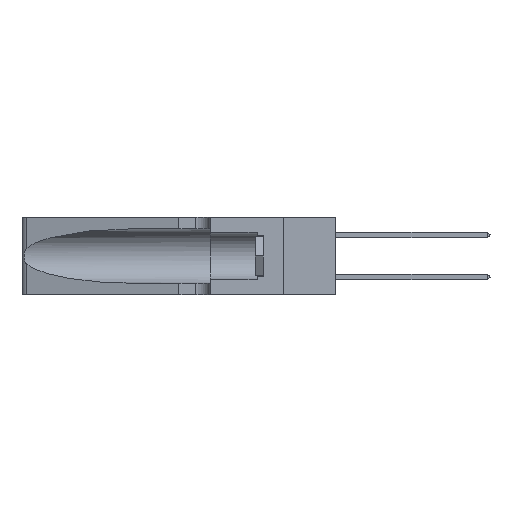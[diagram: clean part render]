
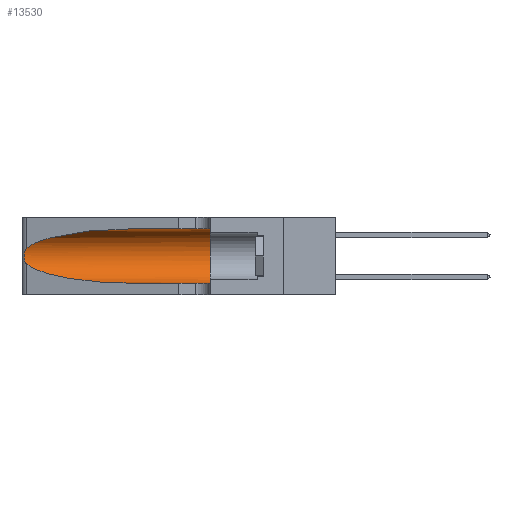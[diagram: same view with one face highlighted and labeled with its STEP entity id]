
A CAD part, left-side view. The second image highlights one B-rep face of the part: STEP entity #13530.
In plain terms, the highlighted cylindrical face has radius 3.308 mm (diameter 6.617 mm), a partial arc.
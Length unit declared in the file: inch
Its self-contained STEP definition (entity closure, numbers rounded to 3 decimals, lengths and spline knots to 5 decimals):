
#371 = CARTESIAN_POINT ( 'NONE',  ( 0.25487, 1.22718, 0.14631 ) ) ;
#1066 = CARTESIAN_POINT ( 'NONE',  ( 0.1305, 0.35, 0.185 ) ) ;
#2398 = CARTESIAN_POINT ( 'NONE',  ( 0.25487, 1.22718, 0.14631 ) ) ;
#3431 = ORIENTED_EDGE ( 'NONE', *, *, #36711, .T. ) ;
#3549 = VERTEX_POINT ( 'NONE', #10067 ) ;
#3583 = CARTESIAN_POINT ( 'NONE',  ( 0.18966, 0.96281, 0.05475 ) ) ;
#4281 = DIRECTION ( 'NONE',  ( 0., 0., 1. ) ) ;
#5246 = CARTESIAN_POINT ( 'NONE',  ( 0.25787, 1.23484, 0.2124 ) ) ;
#6549 = AXIS2_PLACEMENT_3D ( 'NONE', #31095, #12127, #34267 ) ;
#7136 =( BOUNDED_CURVE ( )  B_SPLINE_CURVE ( 3, ( #371, #22571, #3583, #25763 ),
 .UNSPECIFIED., .F., .F. ) 
 B_SPLINE_CURVE_WITH_KNOTS ( ( 4, 4 ),
 ( 3.44316, 4.71239 ),
 .UNSPECIFIED. ) 
 CURVE ( )  GEOMETRIC_REPRESENTATION_ITEM ( )  RATIONAL_B_SPLINE_CURVE ( ( 1., 0.87, 0.87, 1. ) ) 
 REPRESENTATION_ITEM ( '' )  );
#7374 = CARTESIAN_POINT ( 'NONE',  ( 0.18966, 0.96281, 0.31525 ) ) ;
#7692 = VERTEX_POINT ( 'NONE', #39892 ) ;
#8450 = CARTESIAN_POINT ( 'NONE',  ( 0.26018, 1.23835, 0.19895 ) ) ;
#10067 = CARTESIAN_POINT ( 'NONE',  ( 0.1305, 0.35, 0.31525 ) ) ;
#10235 = EDGE_CURVE ( 'NONE', #15838, #3549, #18555, .T. ) ;
#10703 = CARTESIAN_POINT ( 'NONE',  ( 0.25487, 1.22718, 0.22369 ) ) ;
#11637 = CARTESIAN_POINT ( 'NONE',  ( 0.26075, 1.23896, 0.178 ) ) ;
#12127 = DIRECTION ( 'NONE',  ( 0., -1., 0. ) ) ;
#12201 = ORIENTED_EDGE ( 'NONE', *, *, #10235, .F. ) ;
#12465 = EDGE_CURVE ( 'NONE', #3549, #7692, #32204, .T. ) ;
#12592 = CARTESIAN_POINT ( 'NONE',  ( 0.1305, 0.72297, 0.05475 ) ) ;
#13333 = EDGE_CURVE ( 'NONE', #40776, #7692, #33110, .T. ) ;
#13474 = CARTESIAN_POINT ( 'NONE',  ( 0.1305, 1.61858, 0.31525 ) ) ;
#13530 = ADVANCED_FACE ( 'NONE', ( #17751 ), #33596, .F. ) ;
#13596 = ORIENTED_EDGE ( 'NONE', *, *, #12465, .F. ) ;
#14539 =( BOUNDED_CURVE ( )  B_SPLINE_CURVE ( 3, ( #32715, #7374, #29679, #10703 ),
 .UNSPECIFIED., .F., .F. ) 
 B_SPLINE_CURVE_WITH_KNOTS ( ( 4, 4 ),
 ( 1.5708, 2.84003 ),
 .UNSPECIFIED. ) 
 CURVE ( )  GEOMETRIC_REPRESENTATION_ITEM ( )  RATIONAL_B_SPLINE_CURVE ( ( 1., 0.87, 0.87, 1. ) ) 
 REPRESENTATION_ITEM ( '' )  );
#14837 = CARTESIAN_POINT ( 'NONE',  ( 0.25856, 1.23593, 0.16098 ) ) ;
#15320 = AXIS2_PLACEMENT_3D ( 'NONE', #1066, #23251, #4281 ) ;
#15533 = CARTESIAN_POINT ( 'NONE',  ( 0.25487, 1.22718, 0.22369 ) ) ;
#15838 = VERTEX_POINT ( 'NONE', #24839 ) ;
#16656 = DIRECTION ( 'NONE',  ( 0., -1., 0. ) ) ;
#17751 = FACE_OUTER_BOUND ( 'NONE', #33322, .T. ) ;
#17870 = CARTESIAN_POINT ( 'NONE',  ( 0.25487, 1.22718, 0.22369 ) ) ;
#18007 = CARTESIAN_POINT ( 'NONE',  ( 0.25639, 1.23186, 0.15144 ) ) ;
#18555 = LINE ( 'NONE', #13474, #33391 ) ;
#20905 = ORIENTED_EDGE ( 'NONE', *, *, #35336, .T. ) ;
#21173 = CARTESIAN_POINT ( 'NONE',  ( 0.25487, 1.22718, 0.14631 ) ) ;
#22571 = CARTESIAN_POINT ( 'NONE',  ( 0.2373, 1.15595, 0.08982 ) ) ;
#23251 = DIRECTION ( 'NONE',  ( 0., 1., 0. ) ) ;
#23894 = DIRECTION ( 'NONE',  ( 0., -1., 0. ) ) ;
#24214 = CARTESIAN_POINT ( 'NONE',  ( 0.25639, 1.23184, 0.21858 ) ) ;
#24839 = CARTESIAN_POINT ( 'NONE',  ( 0.1305, 0.72297, 0.31525 ) ) ;
#25031 = VERTEX_POINT ( 'NONE', #15533 ) ;
#25763 = CARTESIAN_POINT ( 'NONE',  ( 0.1305, 0.72297, 0.05475 ) ) ;
#27421 = CARTESIAN_POINT ( 'NONE',  ( 0.25854, 1.2359, 0.20912 ) ) ;
#29679 = CARTESIAN_POINT ( 'NONE',  ( 0.2373, 1.15595, 0.28018 ) ) ;
#30607 = CARTESIAN_POINT ( 'NONE',  ( 0.26075, 1.23896, 0.19203 ) ) ;
#31095 = CARTESIAN_POINT ( 'NONE',  ( 0.1305, 1.61858, 0.185 ) ) ;
#32122 = VECTOR ( 'NONE', #23894, 39.37008 ) ;
#32204 = CIRCLE ( 'NONE', #15320, 0.13025 ) ;
#32715 = CARTESIAN_POINT ( 'NONE',  ( 0.1305, 0.72297, 0.31525 ) ) ;
#33110 = LINE ( 'NONE', #39652, #32122 ) ;
#33322 = EDGE_LOOP ( 'NONE', ( #20905, #39458, #3431, #34044, #13596, #12201 ) ) ;
#33391 = VECTOR ( 'NONE', #16656, 39.37008 ) ;
#33596 = CYLINDRICAL_SURFACE ( 'NONE', #6549, 0.13025 ) ;
#33635 = CARTESIAN_POINT ( 'NONE',  ( 0.25555, 1.22994, 0.2215 ) ) ;
#33779 = CARTESIAN_POINT ( 'NONE',  ( 0.26017, 1.23833, 0.17102 ) ) ;
#34044 = ORIENTED_EDGE ( 'NONE', *, *, #13333, .T. ) ;
#34267 = DIRECTION ( 'NONE',  ( 0., 0., -1. ) ) ;
#34935 = VERTEX_POINT ( 'NONE', #2398 ) ;
#35336 = EDGE_CURVE ( 'NONE', #15838, #25031, #14539, .T. ) ;
#36711 = EDGE_CURVE ( 'NONE', #34935, #40776, #7136, .T. ) ;
#36960 = CARTESIAN_POINT ( 'NONE',  ( 0.25789, 1.23486, 0.15765 ) ) ;
#38961 = EDGE_CURVE ( 'NONE', #25031, #34935, #40843, .T. ) ;
#39458 = ORIENTED_EDGE ( 'NONE', *, *, #38961, .T. ) ;
#39652 = CARTESIAN_POINT ( 'NONE',  ( 0.1305, 1.61858, 0.05475 ) ) ;
#39892 = CARTESIAN_POINT ( 'NONE',  ( 0.1305, 0.35, 0.05475 ) ) ;
#40106 = CARTESIAN_POINT ( 'NONE',  ( 0.25555, 1.22993, 0.14849 ) ) ;
#40776 = VERTEX_POINT ( 'NONE', #12592 ) ;
#40843 = B_SPLINE_CURVE_WITH_KNOTS ( 'NONE', 3,
 ( #17870, #33635, #24214, #5246, #27421, #8450, #30607, #11637, #33779, #14837, #36960, #18007, #40106, #21173 ),
 .UNSPECIFIED., .F., .F.,
 ( 4, 2, 2, 2, 2, 2, 4 ),
 ( 0., 0.00027, 0.00053, 0.00107, 0.0016, 0.00187, 0.00214 ),
 .UNSPECIFIED. ) ;
